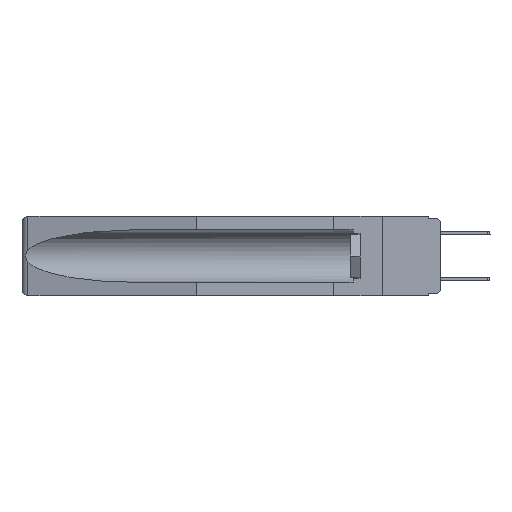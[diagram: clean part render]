
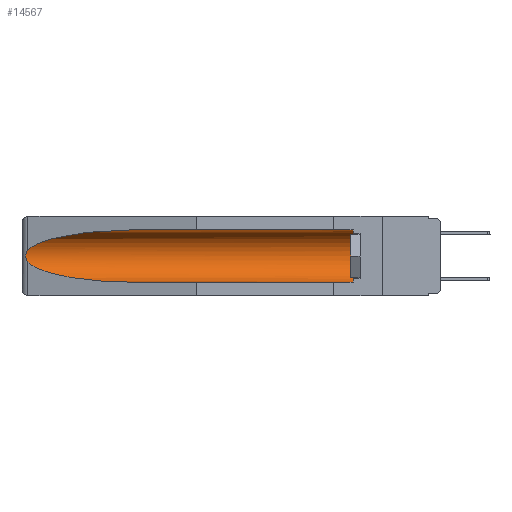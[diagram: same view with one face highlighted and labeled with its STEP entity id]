
A CAD part, left-side view. The second image highlights one B-rep face of the part: STEP entity #14567.
In plain terms, the highlighted cylindrical face has radius 2.857 mm (diameter 5.715 mm), a partial arc.
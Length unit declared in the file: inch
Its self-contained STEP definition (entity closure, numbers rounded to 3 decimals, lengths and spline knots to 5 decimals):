
#537 = CARTESIAN_POINT ( 'NONE',  ( 0.155, -0.30754, -0.059 ) ) ;
#627 = CARTESIAN_POINT ( 'NONE',  ( 0.155, -0.30754, -0.284 ) ) ;
#831 = CARTESIAN_POINT ( 'NONE',  ( 0.25451, 1.48313, -0.09465 ) ) ;
#1021 = CARTESIAN_POINT ( 'NONE',  ( 0.26537, 1.52718, -0.14972 ) ) ;
#1646 = VECTOR ( 'NONE', #26968, 39.37008 ) ;
#1968 = CARTESIAN_POINT ( 'NONE',  ( 0.155, 1.07973, -0.284 ) ) ;
#2804 = CARTESIAN_POINT ( 'NONE',  ( 0.26537, 1.52718, -0.14972 ) ) ;
#2910 = DIRECTION ( 'NONE',  ( 0., -1., 0. ) ) ;
#3387 = CARTESIAN_POINT ( 'NONE',  ( 0.2675, 1.53308, -0.17534 ) ) ;
#3586 = EDGE_CURVE ( 'NONE', #20558, #5397, #20162, .T. ) ;
#3696 = EDGE_CURVE ( 'NONE', #21057, #20536, #17415, .T. ) ;
#3889 =( BOUNDED_CURVE ( )  B_SPLINE_CURVE ( 3, ( #26787, #20328, #831, #24682 ),
 .UNSPECIFIED., .F., .F. ) 
 B_SPLINE_CURVE_WITH_KNOTS ( ( 4, 4 ),
 ( 4.71239, 6.08839 ),
 .UNSPECIFIED. ) 
 CURVE ( )  GEOMETRIC_REPRESENTATION_ITEM ( )  RATIONAL_B_SPLINE_CURVE ( ( 1., 0.848, 0.848, 1. ) ) 
 REPRESENTATION_ITEM ( '' )  );
#4749 = B_SPLINE_CURVE_WITH_KNOTS ( 'NONE', 3,
 ( #2804, #12105, #5591, #27207, #25018, #3387, #20846, #14082, #27123, #24915 ),
 .UNSPECIFIED., .F., .F.,
 ( 4, 2, 2, 2, 4 ),
 ( 0., 0.00029, 0.00058, 0.00087, 0.00117 ),
 .UNSPECIFIED. ) ;
#5170 = CARTESIAN_POINT ( 'NONE',  ( 0.155, -0.30754, -0.1715 ) ) ;
#5198 = AXIS2_PLACEMENT_3D ( 'NONE', #5170, #7462, #20430 ) ;
#5397 = VERTEX_POINT ( 'NONE', #17613 ) ;
#5471 = ORIENTED_EDGE ( 'NONE', *, *, #3696, .T. ) ;
#5591 = CARTESIAN_POINT ( 'NONE',  ( 0.26654, 1.53092, -0.15636 ) ) ;
#5742 = AXIS2_PLACEMENT_3D ( 'NONE', #24827, #2910, #20194 ) ;
#7408 = LINE ( 'NONE', #627, #8766 ) ;
#7462 = DIRECTION ( 'NONE',  ( 0., 1., 0. ) ) ;
#7803 = EDGE_LOOP ( 'NONE', ( #13809, #10934, #10588, #11262, #12302, #5471 ) ) ;
#7954 = CYLINDRICAL_SURFACE ( 'NONE', #5198, 0.1125 ) ;
#8766 = VECTOR ( 'NONE', #13659, 39.37008 ) ;
#10588 = ORIENTED_EDGE ( 'NONE', *, *, #3586, .T. ) ;
#10934 = ORIENTED_EDGE ( 'NONE', *, *, #23386, .T. ) ;
#10984 = EDGE_CURVE ( 'NONE', #20536, #15703, #3889, .T. ) ;
#11262 = ORIENTED_EDGE ( 'NONE', *, *, #20792, .F. ) ;
#12105 = CARTESIAN_POINT ( 'NONE',  ( 0.26597, 1.52961, -0.15275 ) ) ;
#12302 = ORIENTED_EDGE ( 'NONE', *, *, #21380, .T. ) ;
#13659 = DIRECTION ( 'NONE',  ( 0., 1., 0. ) ) ;
#13809 = ORIENTED_EDGE ( 'NONE', *, *, #10984, .T. ) ;
#14082 = CARTESIAN_POINT ( 'NONE',  ( 0.26655, 1.53094, -0.18657 ) ) ;
#14567 = ADVANCED_FACE ( 'NONE', ( #21607 ), #7954, .F. ) ;
#14991 = CARTESIAN_POINT ( 'NONE',  ( 0.26537, 1.52718, -0.19328 ) ) ;
#15064 = CARTESIAN_POINT ( 'NONE',  ( 0.25451, 1.48313, -0.24835 ) ) ;
#15703 = VERTEX_POINT ( 'NONE', #1021 ) ;
#16953 = CIRCLE ( 'NONE', #5742, 0.1125 ) ;
#17415 = LINE ( 'NONE', #537, #1646 ) ;
#17613 = CARTESIAN_POINT ( 'NONE',  ( 0.155, 1.07973, -0.284 ) ) ;
#19473 = CARTESIAN_POINT ( 'NONE',  ( 0.155, 1.07973, -0.059 ) ) ;
#20162 =( BOUNDED_CURVE ( )  B_SPLINE_CURVE ( 3, ( #25905, #15064, #23150, #1968 ),
 .UNSPECIFIED., .F., .F. ) 
 B_SPLINE_CURVE_WITH_KNOTS ( ( 4, 4 ),
 ( 0.1948, 1.5708 ),
 .UNSPECIFIED. ) 
 CURVE ( )  GEOMETRIC_REPRESENTATION_ITEM ( )  RATIONAL_B_SPLINE_CURVE ( ( 1., 0.848, 0.848, 1. ) ) 
 REPRESENTATION_ITEM ( '' )  );
#20194 = DIRECTION ( 'NONE',  ( 0., 0., 1. ) ) ;
#20328 = CARTESIAN_POINT ( 'NONE',  ( 0.21114, 1.30732, -0.059 ) ) ;
#20430 = DIRECTION ( 'NONE',  ( 0., 0., 1. ) ) ;
#20536 = VERTEX_POINT ( 'NONE', #19473 ) ;
#20558 = VERTEX_POINT ( 'NONE', #14991 ) ;
#20792 = EDGE_CURVE ( 'NONE', #23676, #5397, #7408, .T. ) ;
#20846 = CARTESIAN_POINT ( 'NONE',  ( 0.2673, 1.53269, -0.17917 ) ) ;
#21057 = VERTEX_POINT ( 'NONE', #21256 ) ;
#21256 = CARTESIAN_POINT ( 'NONE',  ( 0.155, 0.126, -0.059 ) ) ;
#21380 = EDGE_CURVE ( 'NONE', #23676, #21057, #16953, .T. ) ;
#21607 = FACE_OUTER_BOUND ( 'NONE', #7803, .T. ) ;
#23150 = CARTESIAN_POINT ( 'NONE',  ( 0.21114, 1.30732, -0.284 ) ) ;
#23386 = EDGE_CURVE ( 'NONE', #15703, #20558, #4749, .T. ) ;
#23676 = VERTEX_POINT ( 'NONE', #25881 ) ;
#24682 = CARTESIAN_POINT ( 'NONE',  ( 0.26537, 1.52718, -0.14972 ) ) ;
#24827 = CARTESIAN_POINT ( 'NONE',  ( 0.155, 0.126, -0.1715 ) ) ;
#24915 = CARTESIAN_POINT ( 'NONE',  ( 0.26537, 1.52718, -0.19328 ) ) ;
#25018 = CARTESIAN_POINT ( 'NONE',  ( 0.2675, 1.53308, -0.16763 ) ) ;
#25881 = CARTESIAN_POINT ( 'NONE',  ( 0.155, 0.126, -0.284 ) ) ;
#25905 = CARTESIAN_POINT ( 'NONE',  ( 0.26537, 1.52718, -0.19328 ) ) ;
#26787 = CARTESIAN_POINT ( 'NONE',  ( 0.155, 1.07973, -0.059 ) ) ;
#26968 = DIRECTION ( 'NONE',  ( 0., 1., 0. ) ) ;
#27123 = CARTESIAN_POINT ( 'NONE',  ( 0.26597, 1.5296, -0.19026 ) ) ;
#27207 = CARTESIAN_POINT ( 'NONE',  ( 0.2673, 1.5327, -0.16383 ) ) ;
